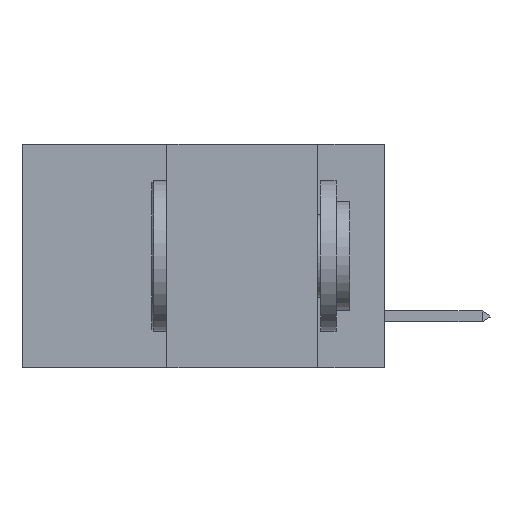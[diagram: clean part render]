
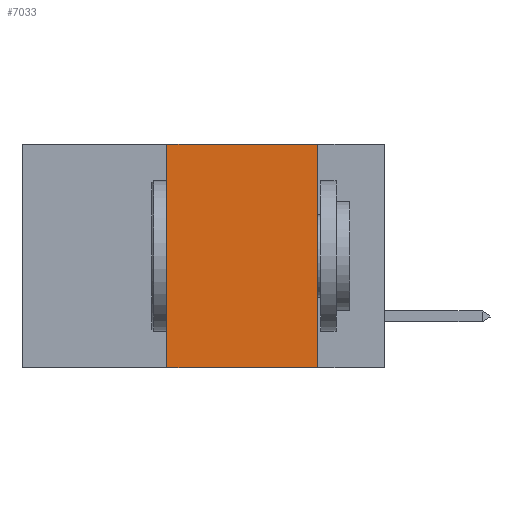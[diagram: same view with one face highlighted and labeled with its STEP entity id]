
A CAD part, left-side view. The second image highlights one B-rep face of the part: STEP entity #7033.
In plain terms, the highlighted planar face has unit normal (-1, 0, 0).
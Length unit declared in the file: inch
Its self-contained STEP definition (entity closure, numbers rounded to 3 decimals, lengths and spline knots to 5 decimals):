
#345 = DIRECTION ( 'NONE',  ( 0., 0., -1. ) ) ;
#468 = CARTESIAN_POINT ( 'NONE',  ( 0., 0.11, 0. ) ) ;
#936 = CARTESIAN_POINT ( 'NONE',  ( 0., 0.36, -0.37 ) ) ;
#2859 = CARTESIAN_POINT ( 'NONE',  ( 0., 0.6, 0. ) ) ;
#3146 = LINE ( 'NONE', #2859, #18847 ) ;
#3466 = CARTESIAN_POINT ( 'NONE',  ( 0., 0.36, 0. ) ) ;
#4159 = DIRECTION ( 'NONE',  ( 0., 0., -1. ) ) ;
#4267 = ORIENTED_EDGE ( 'NONE', *, *, #10726, .T. ) ;
#4904 = VERTEX_POINT ( 'NONE', #936 ) ;
#5237 = VERTEX_POINT ( 'NONE', #468 ) ;
#6150 = VECTOR ( 'NONE', #11852, 39.37008 ) ;
#7033 = ADVANCED_FACE ( 'NONE', ( #25188 ), #9359, .F. ) ;
#7339 = VERTEX_POINT ( 'NONE', #3466 ) ;
#8085 = CARTESIAN_POINT ( 'NONE',  ( 0., 0.11, 0. ) ) ;
#8329 = ORIENTED_EDGE ( 'NONE', *, *, #20565, .F. ) ;
#8872 = CARTESIAN_POINT ( 'NONE',  ( 0., 0.6, -0.37 ) ) ;
#9359 = PLANE ( 'NONE',  #15015 ) ;
#9391 = VERTEX_POINT ( 'NONE', #12155 ) ;
#9685 = LINE ( 'NONE', #8085, #12068 ) ;
#10726 = EDGE_CURVE ( 'NONE', #4904, #9391, #31585, .T. ) ;
#11405 = DIRECTION ( 'NONE',  ( 0., -1., 0. ) ) ;
#11852 = DIRECTION ( 'NONE',  ( 0., 0., 1. ) ) ;
#12068 = VECTOR ( 'NONE', #345, 39.37008 ) ;
#12155 = CARTESIAN_POINT ( 'NONE',  ( 0., 0.11, -0.37 ) ) ;
#12464 = LINE ( 'NONE', #31824, #6150 ) ;
#13078 = DIRECTION ( 'NONE',  ( 0., -1., 0. ) ) ;
#15015 = AXIS2_PLACEMENT_3D ( 'NONE', #21500, #24436, #4159 ) ;
#18847 = VECTOR ( 'NONE', #13078, 39.37008 ) ;
#19835 = EDGE_LOOP ( 'NONE', ( #8329, #27701, #21525, #4267 ) ) ;
#20565 = EDGE_CURVE ( 'NONE', #5237, #9391, #9685, .T. ) ;
#21500 = CARTESIAN_POINT ( 'NONE',  ( 0., 0.6, 0. ) ) ;
#21525 = ORIENTED_EDGE ( 'NONE', *, *, #21541, .F. ) ;
#21541 = EDGE_CURVE ( 'NONE', #4904, #7339, #12464, .T. ) ;
#24436 = DIRECTION ( 'NONE',  ( 1., 0., 0. ) ) ;
#25188 = FACE_OUTER_BOUND ( 'NONE', #19835, .T. ) ;
#27701 = ORIENTED_EDGE ( 'NONE', *, *, #28617, .F. ) ;
#28617 = EDGE_CURVE ( 'NONE', #7339, #5237, #3146, .T. ) ;
#30021 = VECTOR ( 'NONE', #11405, 39.37008 ) ;
#31585 = LINE ( 'NONE', #8872, #30021 ) ;
#31824 = CARTESIAN_POINT ( 'NONE',  ( 0., 0.36, 0. ) ) ;
